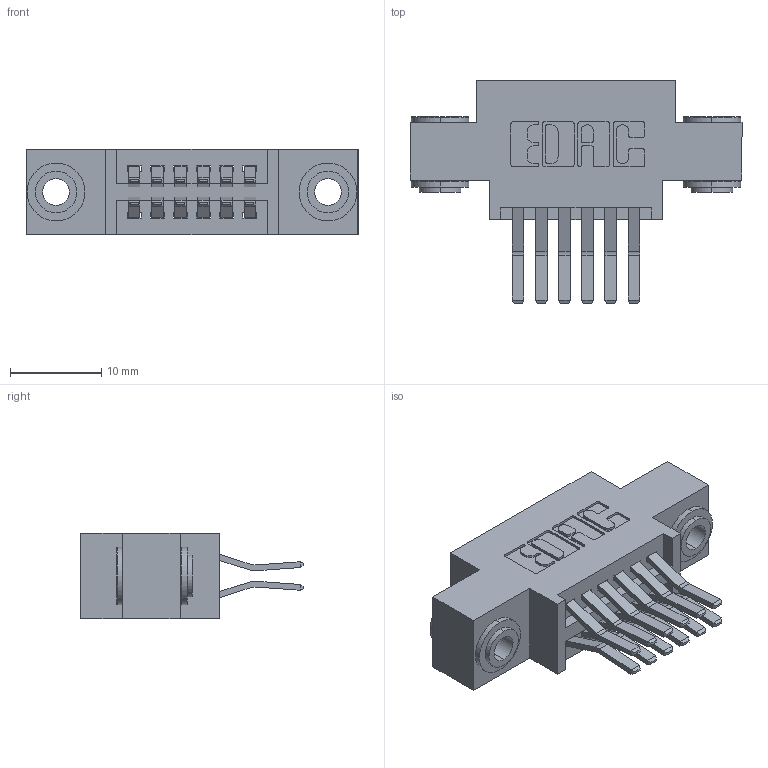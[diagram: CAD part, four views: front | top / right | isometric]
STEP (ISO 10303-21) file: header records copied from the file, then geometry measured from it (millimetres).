
FILE_DESCRIPTION (( 'STEP AP203' ), '1' );
FILE_NAME ('395-012-560-803.STEP', '2018-11-05T20:23:49', ( '' ), ( '' ), 'SwSTEP 2.0', 'SolidWorks 2016', '' );
FILE_SCHEMA (( 'CONFIG_CONTROL_DESIGN' ));
Length unit declared in the file: inch
Products named in the file (4): 395-012-560-803; 345 Part_0.170 Offset - 0.156 Dia-TH; 345-250-002_345-250-002-102; 345-292-001_560 Tail
Assembly tree (15 placements, depth 2):
  395-012-560-803
    345 Part_0.170 Offset - 0.156 Dia-TH
    345-292-001_560 Tail  x12
    345-250-002_345-250-002-102  x2
Bounding box: 36.45 x 24.45 x 9.4 mm (x, y, z)
Volume: 3191.2 mm3; surface area: 4570.5 mm2
Topology: 15 solids, 15 shells, 792 faces, 2289 edges, 1506 vertices
Faces by surface type: plane 490, cylinder 294, cone 8
Entity records: 10424 total; most frequent: CARTESIAN_POINT 1759, ORIENTED_EDGE 1686, DIRECTION 1629, EDGE_CURVE 843, LINE 659, VECTOR 659, VERTEX_POINT 558, AXIS2_PLACEMENT_3D 485
